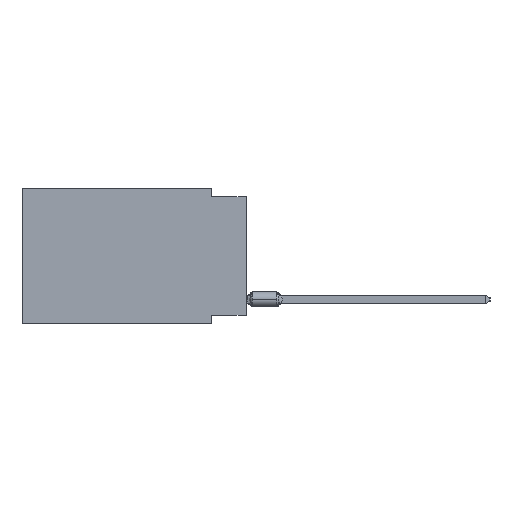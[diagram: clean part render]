
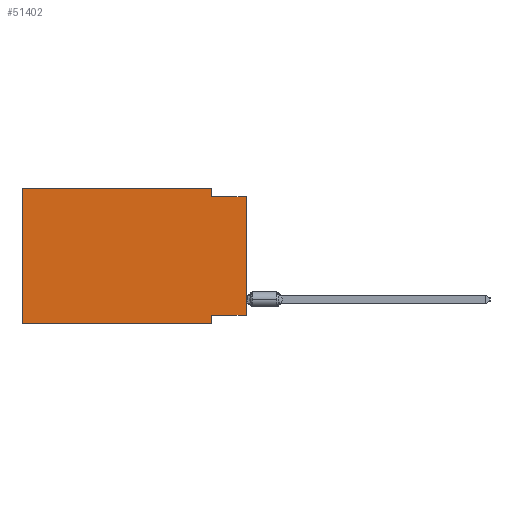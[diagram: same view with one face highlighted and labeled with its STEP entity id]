
A CAD part, left-side view. The second image highlights one B-rep face of the part: STEP entity #51402.
In plain terms, the highlighted planar face has unit normal (-1, 0, 0).
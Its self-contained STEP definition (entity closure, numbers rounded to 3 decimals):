
#296 = EDGE_CURVE ( 'NONE', #42444, #20082, #16177, .T. ) ;
#2206 = CARTESIAN_POINT ( 'NONE',  ( 0., 0., -9.271 ) ) ;
#3880 = ORIENTED_EDGE ( 'NONE', *, *, #17517, .T. ) ;
#7559 = PLANE ( 'NONE',  #22042 ) ;
#7865 = CARTESIAN_POINT ( 'NONE',  ( 0., 2.54, -9.271 ) ) ;
#7989 = LINE ( 'NONE', #33940, #35601 ) ;
#11144 = VECTOR ( 'NONE', #21151, 1000. ) ;
#12189 = ORIENTED_EDGE ( 'NONE', *, *, #20622, .F. ) ;
#12907 = VERTEX_POINT ( 'NONE', #30453 ) ;
#13730 = CARTESIAN_POINT ( 'NONE',  ( 0., 2.54, -9.906 ) ) ;
#14076 = VECTOR ( 'NONE', #25797, 1000. ) ;
#15459 = VECTOR ( 'NONE', #30558, 1000. ) ;
#16177 = LINE ( 'NONE', #20365, #31396 ) ;
#16614 = VERTEX_POINT ( 'NONE', #7865 ) ;
#16712 = EDGE_LOOP ( 'NONE', ( #3880, #24621, #31202, #30111, #44832, #53325, #12189, #26005 ) ) ;
#16978 = CARTESIAN_POINT ( 'NONE',  ( 0., 2.54, -9.906 ) ) ;
#17246 = VECTOR ( 'NONE', #36691, 1000. ) ;
#17517 = EDGE_CURVE ( 'NONE', #47605, #12907, #7989, .T. ) ;
#17992 = LINE ( 'NONE', #48162, #15459 ) ;
#19003 = FACE_OUTER_BOUND ( 'NONE', #16712, .T. ) ;
#19364 = CARTESIAN_POINT ( 'NONE',  ( 0., 16.383, 0. ) ) ;
#20082 = VERTEX_POINT ( 'NONE', #28776 ) ;
#20365 = CARTESIAN_POINT ( 'NONE',  ( 0., 2.54, 0. ) ) ;
#20622 = EDGE_CURVE ( 'NONE', #16614, #43664, #42403, .T. ) ;
#21151 = DIRECTION ( 'NONE',  ( 0., 0., -1. ) ) ;
#21757 = EDGE_CURVE ( 'NONE', #50483, #42444, #43823, .T. ) ;
#22042 = AXIS2_PLACEMENT_3D ( 'NONE', #50031, #24309, #44990 ) ;
#22838 = CARTESIAN_POINT ( 'NONE',  ( 0., 2.54, 0. ) ) ;
#23426 = VECTOR ( 'NONE', #32845, 1000. ) ;
#24309 = DIRECTION ( 'NONE',  ( 1., 0., 0. ) ) ;
#24621 = ORIENTED_EDGE ( 'NONE', *, *, #38470, .F. ) ;
#25001 = LINE ( 'NONE', #42044, #14076 ) ;
#25702 = VERTEX_POINT ( 'NONE', #43061 ) ;
#25797 = DIRECTION ( 'NONE',  ( 0., -1., 0. ) ) ;
#26005 = ORIENTED_EDGE ( 'NONE', *, *, #30321, .F. ) ;
#28663 = LINE ( 'NONE', #37608, #23426 ) ;
#28776 = CARTESIAN_POINT ( 'NONE',  ( 0., 2.54, -0.635 ) ) ;
#30111 = ORIENTED_EDGE ( 'NONE', *, *, #21757, .F. ) ;
#30321 = EDGE_CURVE ( 'NONE', #47605, #16614, #28663, .T. ) ;
#30453 = CARTESIAN_POINT ( 'NONE',  ( 0., 0., -0.635 ) ) ;
#30558 = DIRECTION ( 'NONE',  ( 0., -1., 0. ) ) ;
#31198 = EDGE_CURVE ( 'NONE', #25702, #43664, #17992, .T. ) ;
#31202 = ORIENTED_EDGE ( 'NONE', *, *, #296, .F. ) ;
#31365 = EDGE_CURVE ( 'NONE', #25702, #50483, #44798, .T. ) ;
#31396 = VECTOR ( 'NONE', #33208, 1000. ) ;
#32845 = DIRECTION ( 'NONE',  ( 0., 1., 0. ) ) ;
#33208 = DIRECTION ( 'NONE',  ( 0., 0., -1. ) ) ;
#33940 = CARTESIAN_POINT ( 'NONE',  ( 0., 0., 0. ) ) ;
#35601 = VECTOR ( 'NONE', #46790, 1000. ) ;
#36691 = DIRECTION ( 'NONE',  ( 0., 0., 1. ) ) ;
#37455 = CARTESIAN_POINT ( 'NONE',  ( 0., 16.383, 0. ) ) ;
#37608 = CARTESIAN_POINT ( 'NONE',  ( 0., 0., -9.271 ) ) ;
#38470 = EDGE_CURVE ( 'NONE', #20082, #12907, #25001, .T. ) ;
#38540 = CARTESIAN_POINT ( 'NONE',  ( 0., 16.383, 0. ) ) ;
#42044 = CARTESIAN_POINT ( 'NONE',  ( 0., 0., -0.635 ) ) ;
#42403 = LINE ( 'NONE', #16978, #11144 ) ;
#42444 = VERTEX_POINT ( 'NONE', #22838 ) ;
#43061 = CARTESIAN_POINT ( 'NONE',  ( 0., 16.383, -9.906 ) ) ;
#43664 = VERTEX_POINT ( 'NONE', #13730 ) ;
#43823 = LINE ( 'NONE', #38540, #52841 ) ;
#44798 = LINE ( 'NONE', #19364, #17246 ) ;
#44832 = ORIENTED_EDGE ( 'NONE', *, *, #31365, .F. ) ;
#44990 = DIRECTION ( 'NONE',  ( 0., 0., -1. ) ) ;
#46790 = DIRECTION ( 'NONE',  ( 0., 0., 1. ) ) ;
#47605 = VERTEX_POINT ( 'NONE', #2206 ) ;
#48009 = DIRECTION ( 'NONE',  ( 0., -1., 0. ) ) ;
#48162 = CARTESIAN_POINT ( 'NONE',  ( 0., 16.383, -9.906 ) ) ;
#50031 = CARTESIAN_POINT ( 'NONE',  ( 0., 16.383, 0. ) ) ;
#50483 = VERTEX_POINT ( 'NONE', #37455 ) ;
#51402 = ADVANCED_FACE ( 'NONE', ( #19003 ), #7559, .F. ) ;
#52841 = VECTOR ( 'NONE', #48009, 1000. ) ;
#53325 = ORIENTED_EDGE ( 'NONE', *, *, #31198, .T. ) ;
